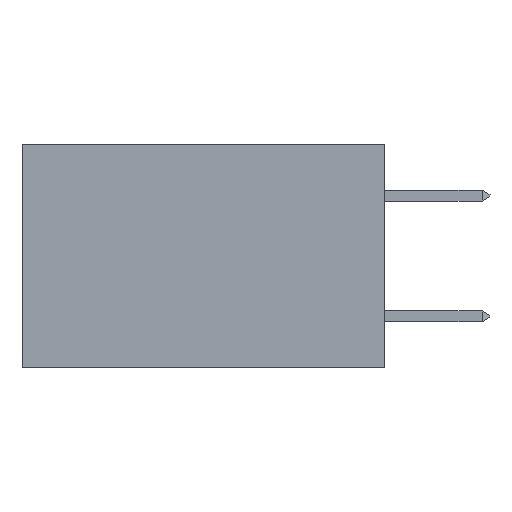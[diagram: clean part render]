
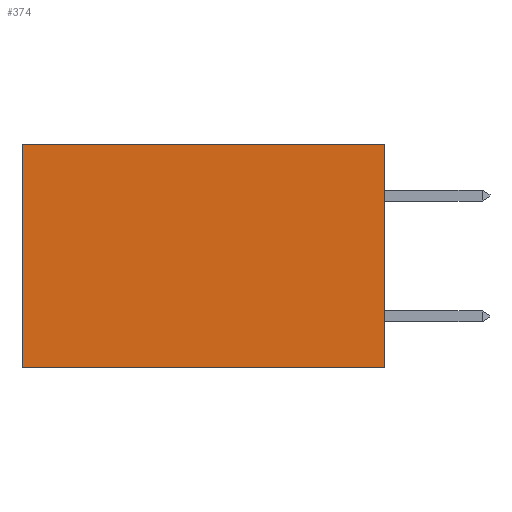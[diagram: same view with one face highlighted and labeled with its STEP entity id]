
A CAD part, left-side view. The second image highlights one B-rep face of the part: STEP entity #374.
In plain terms, the highlighted planar face has unit normal (-1, 0, 0).
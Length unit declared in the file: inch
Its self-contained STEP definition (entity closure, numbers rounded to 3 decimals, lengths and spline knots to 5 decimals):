
#374 = ADVANCED_FACE ( 'NONE', ( #19062 ), #9734, .F. ) ;
#569 = ORIENTED_EDGE ( 'NONE', *, *, #4292, .F. ) ;
#1057 = LINE ( 'NONE', #1476, #10123 ) ;
#1355 = ORIENTED_EDGE ( 'NONE', *, *, #5341, .T. ) ;
#1476 = CARTESIAN_POINT ( 'NONE',  ( 0.2875, 0., -0.37 ) ) ;
#1929 = DIRECTION ( 'NONE',  ( 0., 0., -1. ) ) ;
#2418 = DIRECTION ( 'NONE',  ( 1., 0., 0. ) ) ;
#2858 = EDGE_CURVE ( 'NONE', #12734, #6812, #11827, .T. ) ;
#3238 = DIRECTION ( 'NONE',  ( 0., 0., -1. ) ) ;
#3373 = CARTESIAN_POINT ( 'NONE',  ( 0.2875, 0.6, -0.37 ) ) ;
#3408 = LINE ( 'NONE', #7622, #5266 ) ;
#3931 = DIRECTION ( 'NONE',  ( 0., 0., -1. ) ) ;
#4148 = CARTESIAN_POINT ( 'NONE',  ( 0.2875, 0.6, 0. ) ) ;
#4292 = EDGE_CURVE ( 'NONE', #12734, #7495, #11774, .T. ) ;
#4338 = VERTEX_POINT ( 'NONE', #3373 ) ;
#5221 = EDGE_CURVE ( 'NONE', #7495, #4338, #1057, .T. ) ;
#5266 = VECTOR ( 'NONE', #1929, 39.37008 ) ;
#5341 = EDGE_CURVE ( 'NONE', #6812, #4338, #3408, .T. ) ;
#6156 = DIRECTION ( 'NONE',  ( 0., 1., 0. ) ) ;
#6812 = VERTEX_POINT ( 'NONE', #4148 ) ;
#7495 = VERTEX_POINT ( 'NONE', #10513 ) ;
#7622 = CARTESIAN_POINT ( 'NONE',  ( 0.2875, 0.6, 0. ) ) ;
#8459 = ORIENTED_EDGE ( 'NONE', *, *, #2858, .T. ) ;
#8944 = CARTESIAN_POINT ( 'NONE',  ( 0.2875, 0., 0. ) ) ;
#9734 = PLANE ( 'NONE',  #17747 ) ;
#10123 = VECTOR ( 'NONE', #6156, 39.37008 ) ;
#10513 = CARTESIAN_POINT ( 'NONE',  ( 0.2875, 0., -0.37 ) ) ;
#11774 = LINE ( 'NONE', #8944, #19154 ) ;
#11827 = LINE ( 'NONE', #13644, #13431 ) ;
#12425 = EDGE_LOOP ( 'NONE', ( #1355, #13551, #569, #8459 ) ) ;
#12734 = VERTEX_POINT ( 'NONE', #14278 ) ;
#13431 = VECTOR ( 'NONE', #17919, 39.37008 ) ;
#13551 = ORIENTED_EDGE ( 'NONE', *, *, #5221, .F. ) ;
#13644 = CARTESIAN_POINT ( 'NONE',  ( 0.2875, 0., 0. ) ) ;
#14278 = CARTESIAN_POINT ( 'NONE',  ( 0.2875, 0., 0. ) ) ;
#16982 = CARTESIAN_POINT ( 'NONE',  ( 0.2875, 0., 0. ) ) ;
#17747 = AXIS2_PLACEMENT_3D ( 'NONE', #16982, #2418, #3931 ) ;
#17919 = DIRECTION ( 'NONE',  ( 0., 1., 0. ) ) ;
#19062 = FACE_OUTER_BOUND ( 'NONE', #12425, .T. ) ;
#19154 = VECTOR ( 'NONE', #3238, 39.37008 ) ;
